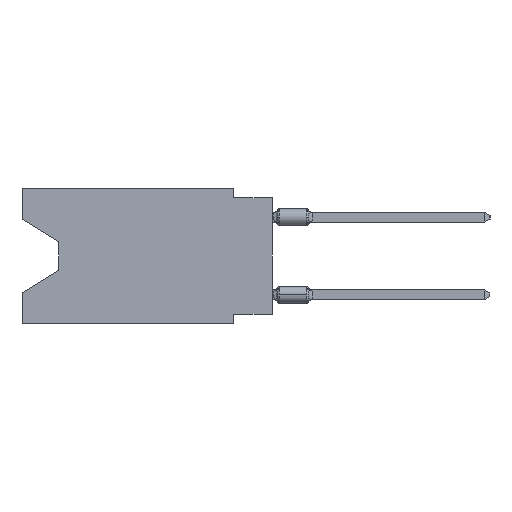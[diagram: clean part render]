
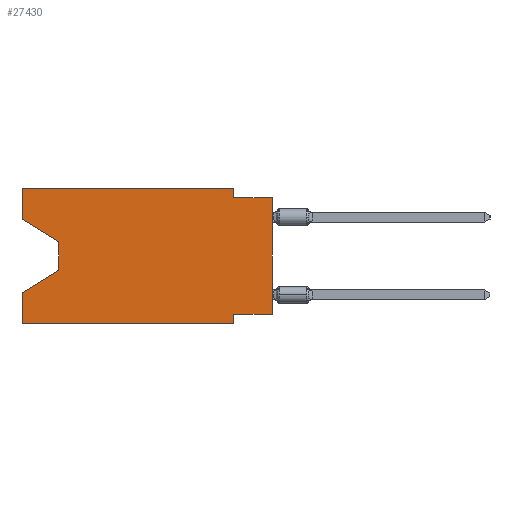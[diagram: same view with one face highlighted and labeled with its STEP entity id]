
A CAD part, left-side view. The second image highlights one B-rep face of the part: STEP entity #27430.
In plain terms, the highlighted planar face has unit normal (-1, 0, 0).
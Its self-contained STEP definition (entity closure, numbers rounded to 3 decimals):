
#185 = VERTEX_POINT ( 'NONE', #59671 ) ;
#1223 = LINE ( 'NONE', #59180, #33294 ) ;
#1640 = LINE ( 'NONE', #40255, #42755 ) ;
#2780 = ORIENTED_EDGE ( 'NONE', *, *, #45350, .F. ) ;
#2898 = DIRECTION ( 'NONE',  ( 0., 0., -1. ) ) ;
#4097 = FACE_OUTER_BOUND ( 'NONE', #14459, .T. ) ;
#4614 = LINE ( 'NONE', #4931, #16103 ) ;
#4931 = CARTESIAN_POINT ( 'NONE',  ( 0., 16.383, -2.038 ) ) ;
#5010 = EDGE_CURVE ( 'NONE', #20096, #44917, #32481, .T. ) ;
#6205 = ORIENTED_EDGE ( 'NONE', *, *, #5010, .F. ) ;
#6206 = DIRECTION ( 'NONE',  ( 0., -1., 0. ) ) ;
#6272 = VERTEX_POINT ( 'NONE', #61409 ) ;
#6698 = CARTESIAN_POINT ( 'NONE',  ( 0., 2.54, 0. ) ) ;
#7954 = LINE ( 'NONE', #26957, #43155 ) ;
#7989 = CARTESIAN_POINT ( 'NONE',  ( 0., 13.97, -5.385 ) ) ;
#8196 = CARTESIAN_POINT ( 'NONE',  ( 0., 0., 0. ) ) ;
#8886 = VECTOR ( 'NONE', #6206, 1000. ) ;
#9717 = VERTEX_POINT ( 'NONE', #6698 ) ;
#10057 = LINE ( 'NONE', #34423, #23293 ) ;
#10112 = VECTOR ( 'NONE', #36371, 1000. ) ;
#12860 = DIRECTION ( 'NONE',  ( 0., 0., 1. ) ) ;
#13247 = DIRECTION ( 'NONE',  ( 0., 0., 1. ) ) ;
#13987 = VECTOR ( 'NONE', #27743, 1000. ) ;
#14459 = EDGE_LOOP ( 'NONE', ( #54091, #62273, #48409, #2780, #34161, #21062, #6205, #26264, #18730, #55741, #26350, #49932 ) ) ;
#16103 = VECTOR ( 'NONE', #57821, 1000. ) ;
#16840 = VERTEX_POINT ( 'NONE', #56766 ) ;
#18730 = ORIENTED_EDGE ( 'NONE', *, *, #48778, .F. ) ;
#19616 = VECTOR ( 'NONE', #13247, 1000. ) ;
#20096 = VERTEX_POINT ( 'NONE', #42916 ) ;
#20880 = EDGE_CURVE ( 'NONE', #26792, #24799, #58575, .T. ) ;
#21062 = ORIENTED_EDGE ( 'NONE', *, *, #52898, .F. ) ;
#21197 = CARTESIAN_POINT ( 'NONE',  ( 0., 16.383, 0. ) ) ;
#21336 = CARTESIAN_POINT ( 'NONE',  ( 0., 0., -0.635 ) ) ;
#22689 = LINE ( 'NONE', #42014, #35855 ) ;
#23293 = VECTOR ( 'NONE', #29364, 1000. ) ;
#24070 = EDGE_CURVE ( 'NONE', #34002, #26792, #1223, .T. ) ;
#24576 = CARTESIAN_POINT ( 'NONE',  ( 0., 16.383, 0. ) ) ;
#24799 = VERTEX_POINT ( 'NONE', #28086 ) ;
#26264 = ORIENTED_EDGE ( 'NONE', *, *, #44930, .T. ) ;
#26350 = ORIENTED_EDGE ( 'NONE', *, *, #30161, .F. ) ;
#26631 = VECTOR ( 'NONE', #54462, 1000. ) ;
#26792 = VERTEX_POINT ( 'NONE', #7989 ) ;
#26957 = CARTESIAN_POINT ( 'NONE',  ( 0., 2.54, -8.89 ) ) ;
#27430 = ADVANCED_FACE ( 'NONE', ( #4097 ), #29098, .F. ) ;
#27448 = CARTESIAN_POINT ( 'NONE',  ( 0., 13.97, -3.505 ) ) ;
#27743 = DIRECTION ( 'NONE',  ( 0., 1., 0. ) ) ;
#28086 = CARTESIAN_POINT ( 'NONE',  ( 0., 16.383, -6.852 ) ) ;
#28436 = VERTEX_POINT ( 'NONE', #57680 ) ;
#29098 = PLANE ( 'NONE',  #46046 ) ;
#29364 = DIRECTION ( 'NONE',  ( 0., 0., -1. ) ) ;
#30161 = EDGE_CURVE ( 'NONE', #16840, #9717, #54050, .T. ) ;
#32481 = LINE ( 'NONE', #51820, #13987 ) ;
#33294 = VECTOR ( 'NONE', #34785, 1000. ) ;
#34002 = VERTEX_POINT ( 'NONE', #27448 ) ;
#34031 = VECTOR ( 'NONE', #53801, 1000. ) ;
#34161 = ORIENTED_EDGE ( 'NONE', *, *, #35812, .T. ) ;
#34423 = CARTESIAN_POINT ( 'NONE',  ( 0., 2.54, 0. ) ) ;
#34785 = DIRECTION ( 'NONE',  ( 0., 0., -1. ) ) ;
#35766 = LINE ( 'NONE', #21197, #10112 ) ;
#35812 = EDGE_CURVE ( 'NONE', #55212, #28436, #41345, .T. ) ;
#35855 = VECTOR ( 'NONE', #12860, 1000. ) ;
#36371 = DIRECTION ( 'NONE',  ( 0., 0., 1. ) ) ;
#37008 = LINE ( 'NONE', #8196, #19616 ) ;
#37981 = DIRECTION ( 'NONE',  ( 0., 0., -1. ) ) ;
#40255 = CARTESIAN_POINT ( 'NONE',  ( 0., 0., -0.635 ) ) ;
#40575 = DIRECTION ( 'NONE',  ( 0., -1., 0. ) ) ;
#41345 = LINE ( 'NONE', #47803, #34031 ) ;
#42014 = CARTESIAN_POINT ( 'NONE',  ( 0., 16.383, 0. ) ) ;
#42746 = DIRECTION ( 'NONE',  ( 1., 0., 0. ) ) ;
#42755 = VECTOR ( 'NONE', #40575, 1000. ) ;
#42916 = CARTESIAN_POINT ( 'NONE',  ( 0., 0., -8.255 ) ) ;
#43155 = VECTOR ( 'NONE', #2898, 1000. ) ;
#44330 = CARTESIAN_POINT ( 'NONE',  ( 0., 13.97, -5.385 ) ) ;
#44917 = VERTEX_POINT ( 'NONE', #56652 ) ;
#44930 = EDGE_CURVE ( 'NONE', #20096, #48320, #37008, .T. ) ;
#45350 = EDGE_CURVE ( 'NONE', #55212, #24799, #22689, .T. ) ;
#46046 = AXIS2_PLACEMENT_3D ( 'NONE', #57303, #42746, #37981 ) ;
#47803 = CARTESIAN_POINT ( 'NONE',  ( 0., 16.383, -8.89 ) ) ;
#48320 = VERTEX_POINT ( 'NONE', #21336 ) ;
#48409 = ORIENTED_EDGE ( 'NONE', *, *, #20880, .T. ) ;
#48778 = EDGE_CURVE ( 'NONE', #185, #48320, #1640, .T. ) ;
#49932 = ORIENTED_EDGE ( 'NONE', *, *, #62318, .F. ) ;
#51820 = CARTESIAN_POINT ( 'NONE',  ( 0., 0., -8.255 ) ) ;
#52898 = EDGE_CURVE ( 'NONE', #44917, #28436, #7954, .T. ) ;
#53801 = DIRECTION ( 'NONE',  ( 0., -1., 0. ) ) ;
#54050 = LINE ( 'NONE', #24576, #8886 ) ;
#54091 = ORIENTED_EDGE ( 'NONE', *, *, #57779, .T. ) ;
#54462 = DIRECTION ( 'NONE',  ( 0., 0.855, -0.519 ) ) ;
#55212 = VERTEX_POINT ( 'NONE', #55600 ) ;
#55600 = CARTESIAN_POINT ( 'NONE',  ( 0., 16.383, -8.89 ) ) ;
#55741 = ORIENTED_EDGE ( 'NONE', *, *, #62560, .F. ) ;
#56652 = CARTESIAN_POINT ( 'NONE',  ( 0., 2.54, -8.255 ) ) ;
#56766 = CARTESIAN_POINT ( 'NONE',  ( 0., 16.383, 0. ) ) ;
#57303 = CARTESIAN_POINT ( 'NONE',  ( 0., 16.383, 0. ) ) ;
#57680 = CARTESIAN_POINT ( 'NONE',  ( 0., 2.54, -8.89 ) ) ;
#57779 = EDGE_CURVE ( 'NONE', #6272, #34002, #4614, .T. ) ;
#57821 = DIRECTION ( 'NONE',  ( 0., -0.855, -0.519 ) ) ;
#58575 = LINE ( 'NONE', #44330, #26631 ) ;
#59180 = CARTESIAN_POINT ( 'NONE',  ( 0., 13.97, -3.505 ) ) ;
#59671 = CARTESIAN_POINT ( 'NONE',  ( 0., 2.54, -0.635 ) ) ;
#61409 = CARTESIAN_POINT ( 'NONE',  ( 0., 16.383, -2.038 ) ) ;
#62273 = ORIENTED_EDGE ( 'NONE', *, *, #24070, .T. ) ;
#62318 = EDGE_CURVE ( 'NONE', #6272, #16840, #35766, .T. ) ;
#62560 = EDGE_CURVE ( 'NONE', #9717, #185, #10057, .T. ) ;
